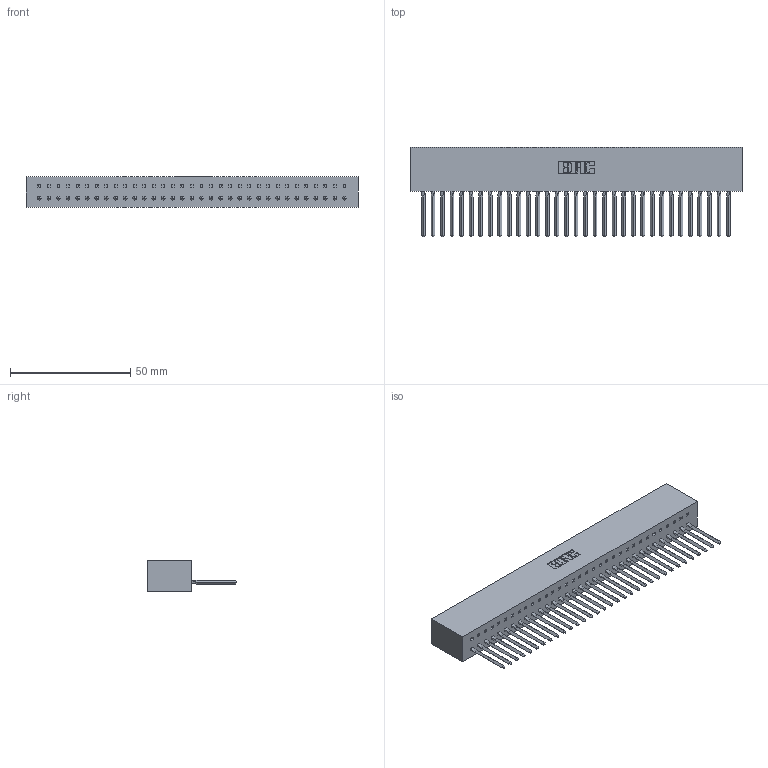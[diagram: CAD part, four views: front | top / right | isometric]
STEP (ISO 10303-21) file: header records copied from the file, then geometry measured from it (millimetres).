
FILE_DESCRIPTION (( 'STEP AP203' ), '1' );
FILE_NAME ('317-033-541-601.STEP', '2020-02-27T21:31:39', ( '' ), ( '' ), 'SwSTEP 2.0', 'SolidWorks 2016', '' );
FILE_SCHEMA (( 'CONFIG_CONTROL_DESIGN' ));
Length unit declared in the file: inch
Products named in the file (3): 317-033-541-601; 317 Part_Lugless; 317-290-002_541
Assembly tree (34 placements, depth 2):
  317-033-541-601
    317 Part_Lugless
    317-290-002_541  x33
Bounding box: 137.97 x 37.34 x 12.7 mm (x, y, z)
Volume: 23803.6 mm3; surface area: 33529.8 mm2
Topology: 34 solids, 34 shells, 5106 faces, 14561 edges, 9464 vertices
Faces by surface type: plane 4142, cylinder 832, bspline 132
Entity records: 49040 total; most frequent: CARTESIAN_POINT 9356, ORIENTED_EDGE 8642, DIRECTION 7083, EDGE_CURVE 4321, LINE 3965, VECTOR 3965, VERTEX_POINT 2872, AXIS2_PLACEMENT_3D 1559
